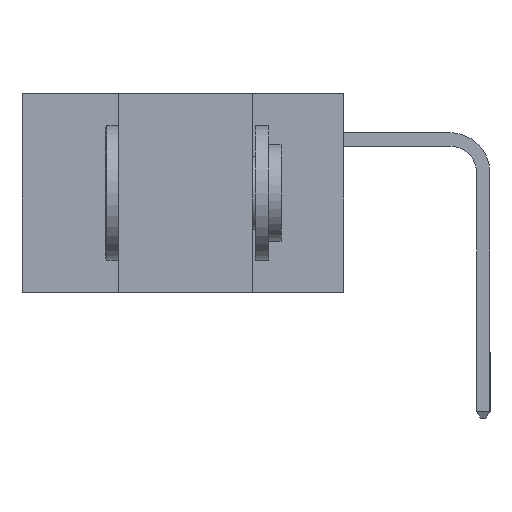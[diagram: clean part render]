
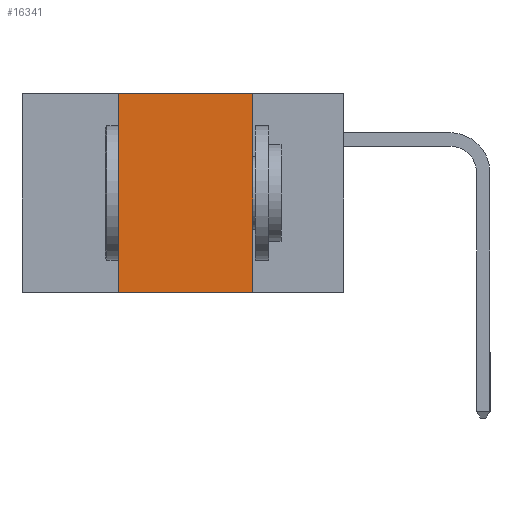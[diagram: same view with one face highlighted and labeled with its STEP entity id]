
A CAD part, left-side view. The second image highlights one B-rep face of the part: STEP entity #16341.
In plain terms, the highlighted planar face has unit normal (-1, 0, 0).
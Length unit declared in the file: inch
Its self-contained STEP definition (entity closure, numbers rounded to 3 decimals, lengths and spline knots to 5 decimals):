
#737 = LINE ( 'NONE', #15985, #6502 ) ;
#862 = CARTESIAN_POINT ( 'NONE',  ( 0., 0.42, -0.37 ) ) ;
#1049 = DIRECTION ( 'NONE',  ( 0., -1., 0. ) ) ;
#1279 = CARTESIAN_POINT ( 'NONE',  ( 0., 0.6, 0. ) ) ;
#2385 = VERTEX_POINT ( 'NONE', #5092 ) ;
#3168 = VECTOR ( 'NONE', #14463, 39.37008 ) ;
#3456 = ORIENTED_EDGE ( 'NONE', *, *, #16995, .F. ) ;
#3810 = CARTESIAN_POINT ( 'NONE',  ( 0., 0.17, -0.37 ) ) ;
#4144 = LINE ( 'NONE', #16066, #3168 ) ;
#4703 = CARTESIAN_POINT ( 'NONE',  ( 0., 0.42, 0. ) ) ;
#5092 = CARTESIAN_POINT ( 'NONE',  ( 0., 0.17, 0. ) ) ;
#5721 = VERTEX_POINT ( 'NONE', #14015 ) ;
#6502 = VECTOR ( 'NONE', #10954, 39.37008 ) ;
#6746 = FACE_OUTER_BOUND ( 'NONE', #22620, .T. ) ;
#7702 = DIRECTION ( 'NONE',  ( 0., 0., -1. ) ) ;
#8727 = ORIENTED_EDGE ( 'NONE', *, *, #17444, .F. ) ;
#9541 = PLANE ( 'NONE',  #16741 ) ;
#10954 = DIRECTION ( 'NONE',  ( 0., 0., 1. ) ) ;
#11087 = ORIENTED_EDGE ( 'NONE', *, *, #16211, .T. ) ;
#12875 = LINE ( 'NONE', #3810, #14562 ) ;
#13122 = VECTOR ( 'NONE', #1049, 39.37008 ) ;
#14015 = CARTESIAN_POINT ( 'NONE',  ( 0., 0.17, -0.37 ) ) ;
#14463 = DIRECTION ( 'NONE',  ( 0., -1., 0. ) ) ;
#14562 = VECTOR ( 'NONE', #7702, 39.37008 ) ;
#15985 = CARTESIAN_POINT ( 'NONE',  ( 0., 0.42, -0.37 ) ) ;
#16066 = CARTESIAN_POINT ( 'NONE',  ( 0., 0.6, -0.37 ) ) ;
#16211 = EDGE_CURVE ( 'NONE', #18366, #5721, #4144, .T. ) ;
#16341 = ADVANCED_FACE ( 'NONE', ( #6746 ), #9541, .F. ) ;
#16533 = DIRECTION ( 'NONE',  ( 1., 0., 0. ) ) ;
#16650 = CARTESIAN_POINT ( 'NONE',  ( 0., 0.6, 0. ) ) ;
#16741 = AXIS2_PLACEMENT_3D ( 'NONE', #16650, #16533, #20655 ) ;
#16995 = EDGE_CURVE ( 'NONE', #18366, #17600, #737, .T. ) ;
#17006 = LINE ( 'NONE', #1279, #13122 ) ;
#17444 = EDGE_CURVE ( 'NONE', #2385, #5721, #12875, .T. ) ;
#17600 = VERTEX_POINT ( 'NONE', #4703 ) ;
#17663 = EDGE_CURVE ( 'NONE', #17600, #2385, #17006, .T. ) ;
#18366 = VERTEX_POINT ( 'NONE', #862 ) ;
#19499 = ORIENTED_EDGE ( 'NONE', *, *, #17663, .F. ) ;
#20655 = DIRECTION ( 'NONE',  ( 0., 0., -1. ) ) ;
#22620 = EDGE_LOOP ( 'NONE', ( #8727, #19499, #3456, #11087 ) ) ;
